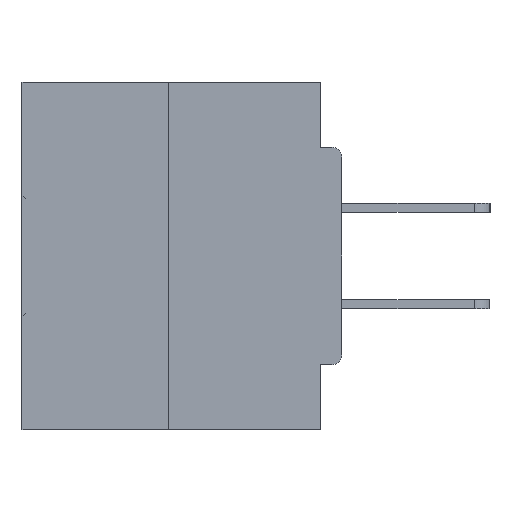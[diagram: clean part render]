
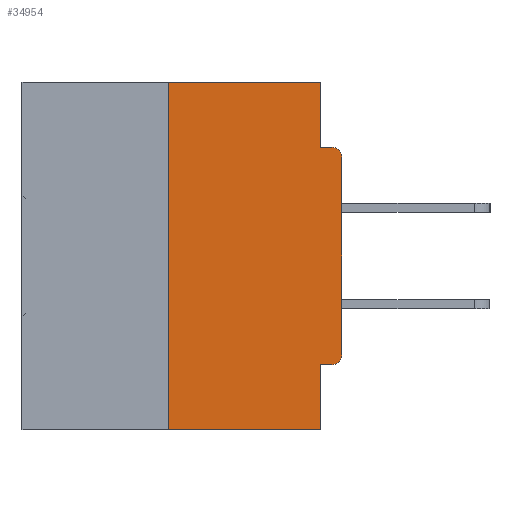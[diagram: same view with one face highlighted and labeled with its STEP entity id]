
A CAD part, left-side view. The second image highlights one B-rep face of the part: STEP entity #34954.
In plain terms, the highlighted planar face has unit normal (-1, 0, 0).
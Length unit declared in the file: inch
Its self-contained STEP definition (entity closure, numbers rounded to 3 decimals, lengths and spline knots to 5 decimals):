
#298 = AXIS2_PLACEMENT_3D ( 'NONE', #41169, #34834, #31178 ) ;
#529 = VECTOR ( 'NONE', #13066, 39.37008 ) ;
#1398 = ORIENTED_EDGE ( 'NONE', *, *, #10693, .T. ) ;
#1466 = ORIENTED_EDGE ( 'NONE', *, *, #30672, .T. ) ;
#1700 = LINE ( 'NONE', #31882, #3762 ) ;
#2365 = EDGE_CURVE ( 'NONE', #16258, #17613, #17728, .T. ) ;
#3525 = VERTEX_POINT ( 'NONE', #18874 ) ;
#3762 = VECTOR ( 'NONE', #38323, 39.37008 ) ;
#4498 = ORIENTED_EDGE ( 'NONE', *, *, #33151, .T. ) ;
#6121 = EDGE_CURVE ( 'NONE', #29353, #7002, #11609, .T. ) ;
#6404 = VERTEX_POINT ( 'NONE', #8780 ) ;
#6416 = ORIENTED_EDGE ( 'NONE', *, *, #14811, .F. ) ;
#7002 = VERTEX_POINT ( 'NONE', #20722 ) ;
#8414 = EDGE_CURVE ( 'NONE', #10260, #23831, #39358, .T. ) ;
#8780 = CARTESIAN_POINT ( 'NONE',  ( 0., 0.031, -0.4065 ) ) ;
#10059 = PLANE ( 'NONE',  #12892 ) ;
#10260 = VERTEX_POINT ( 'NONE', #11143 ) ;
#10693 = EDGE_CURVE ( 'NONE', #39204, #23831, #41880, .T. ) ;
#10961 = DIRECTION ( 'NONE',  ( 0., 0., -1. ) ) ;
#11143 = CARTESIAN_POINT ( 'NONE',  ( 0., 0.031, -0.0935 ) ) ;
#11407 = CARTESIAN_POINT ( 'NONE',  ( 0., 0.031, -0.5 ) ) ;
#11609 = LINE ( 'NONE', #33276, #529 ) ;
#12892 = AXIS2_PLACEMENT_3D ( 'NONE', #13450, #40563, #37018 ) ;
#13066 = DIRECTION ( 'NONE',  ( 0., -1., 0. ) ) ;
#13450 = CARTESIAN_POINT ( 'NONE',  ( 0., 0.46, 0. ) ) ;
#13555 = VECTOR ( 'NONE', #22136, 39.37008 ) ;
#14092 = FACE_OUTER_BOUND ( 'NONE', #43647, .T. ) ;
#14328 = ORIENTED_EDGE ( 'NONE', *, *, #8414, .F. ) ;
#14481 = ORIENTED_EDGE ( 'NONE', *, *, #6121, .F. ) ;
#14692 = CARTESIAN_POINT ( 'NONE',  ( 0., 0., -0.1085 ) ) ;
#14811 = EDGE_CURVE ( 'NONE', #32368, #6404, #1700, .T. ) ;
#15095 = CARTESIAN_POINT ( 'NONE',  ( 0., 0., 0. ) ) ;
#15774 = CARTESIAN_POINT ( 'NONE',  ( 0., 0.015, -0.4065 ) ) ;
#16258 = VERTEX_POINT ( 'NONE', #18510 ) ;
#16690 = EDGE_CURVE ( 'NONE', #7002, #10260, #38430, .T. ) ;
#17613 = VERTEX_POINT ( 'NONE', #38040 ) ;
#17728 = LINE ( 'NONE', #42406, #31461 ) ;
#18332 = LINE ( 'NONE', #38484, #13555 ) ;
#18510 = CARTESIAN_POINT ( 'NONE',  ( 0., 0.25, -0.5 ) ) ;
#18874 = CARTESIAN_POINT ( 'NONE',  ( 0., 0., -0.3915 ) ) ;
#19603 = DIRECTION ( 'NONE',  ( -1., 0., 0. ) ) ;
#20153 = CARTESIAN_POINT ( 'NONE',  ( 0., 0.015, -0.1085 ) ) ;
#20722 = CARTESIAN_POINT ( 'NONE',  ( 0., 0.031, 0. ) ) ;
#21680 = CIRCLE ( 'NONE', #298, 0.015 ) ;
#21708 = EDGE_CURVE ( 'NONE', #6404, #17613, #38833, .T. ) ;
#22136 = DIRECTION ( 'NONE',  ( 0., 0., 1. ) ) ;
#23831 = VERTEX_POINT ( 'NONE', #42630 ) ;
#24298 = CARTESIAN_POINT ( 'NONE',  ( 0., 0., -0.0935 ) ) ;
#24571 = VECTOR ( 'NONE', #10961, 39.37008 ) ;
#25294 = DIRECTION ( 'NONE',  ( 0., -1., 0. ) ) ;
#26825 = EDGE_CURVE ( 'NONE', #16258, #29353, #18332, .T. ) ;
#27733 = DIRECTION ( 'NONE',  ( 0., -1., 0. ) ) ;
#29353 = VERTEX_POINT ( 'NONE', #39860 ) ;
#30370 = VECTOR ( 'NONE', #27733, 39.37008 ) ;
#30672 = EDGE_CURVE ( 'NONE', #32368, #3525, #21680, .T. ) ;
#31178 = DIRECTION ( 'NONE',  ( 0., 0., -1. ) ) ;
#31461 = VECTOR ( 'NONE', #25294, 39.37008 ) ;
#31788 = ORIENTED_EDGE ( 'NONE', *, *, #21708, .F. ) ;
#31882 = CARTESIAN_POINT ( 'NONE',  ( 0., 0., -0.4065 ) ) ;
#32368 = VERTEX_POINT ( 'NONE', #15774 ) ;
#33054 = DIRECTION ( 'NONE',  ( 0., 0., -1. ) ) ;
#33068 = ORIENTED_EDGE ( 'NONE', *, *, #16690, .F. ) ;
#33151 = EDGE_CURVE ( 'NONE', #3525, #39204, #34694, .T. ) ;
#33276 = CARTESIAN_POINT ( 'NONE',  ( 0., 0.46, 0. ) ) ;
#33654 = VECTOR ( 'NONE', #38655, 39.37008 ) ;
#34049 = ORIENTED_EDGE ( 'NONE', *, *, #2365, .T. ) ;
#34694 = LINE ( 'NONE', #15095, #33654 ) ;
#34834 = DIRECTION ( 'NONE',  ( -1., 0., 0. ) ) ;
#34954 = ADVANCED_FACE ( 'NONE', ( #14092 ), #10059, .F. ) ;
#36305 = VECTOR ( 'NONE', #38732, 39.37008 ) ;
#37018 = DIRECTION ( 'NONE',  ( 0., 0., -1. ) ) ;
#37866 = AXIS2_PLACEMENT_3D ( 'NONE', #20153, #19603, #33054 ) ;
#38040 = CARTESIAN_POINT ( 'NONE',  ( 0., 0.031, -0.5 ) ) ;
#38169 = ORIENTED_EDGE ( 'NONE', *, *, #26825, .F. ) ;
#38323 = DIRECTION ( 'NONE',  ( 0., 1., 0. ) ) ;
#38430 = LINE ( 'NONE', #38877, #36305 ) ;
#38484 = CARTESIAN_POINT ( 'NONE',  ( 0., 0.25, 0. ) ) ;
#38655 = DIRECTION ( 'NONE',  ( 0., 0., 1. ) ) ;
#38732 = DIRECTION ( 'NONE',  ( 0., 0., -1. ) ) ;
#38833 = LINE ( 'NONE', #11407, #24571 ) ;
#38877 = CARTESIAN_POINT ( 'NONE',  ( 0., 0.031, 0. ) ) ;
#39204 = VERTEX_POINT ( 'NONE', #14692 ) ;
#39358 = LINE ( 'NONE', #24298, #30370 ) ;
#39860 = CARTESIAN_POINT ( 'NONE',  ( 0., 0.25, 0. ) ) ;
#40563 = DIRECTION ( 'NONE',  ( 1., 0., 0. ) ) ;
#41169 = CARTESIAN_POINT ( 'NONE',  ( 0., 0.015, -0.3915 ) ) ;
#41880 = CIRCLE ( 'NONE', #37866, 0.015 ) ;
#42406 = CARTESIAN_POINT ( 'NONE',  ( 0., 0.46, -0.5 ) ) ;
#42630 = CARTESIAN_POINT ( 'NONE',  ( 0., 0.015, -0.0935 ) ) ;
#43647 = EDGE_LOOP ( 'NONE', ( #14481, #38169, #34049, #31788, #6416, #1466, #4498, #1398, #14328, #33068 ) ) ;
